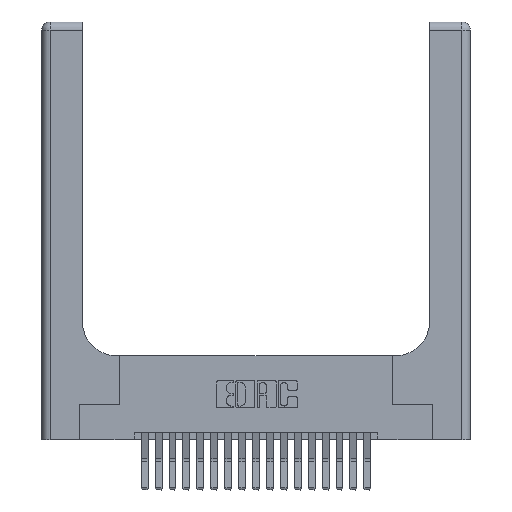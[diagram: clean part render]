
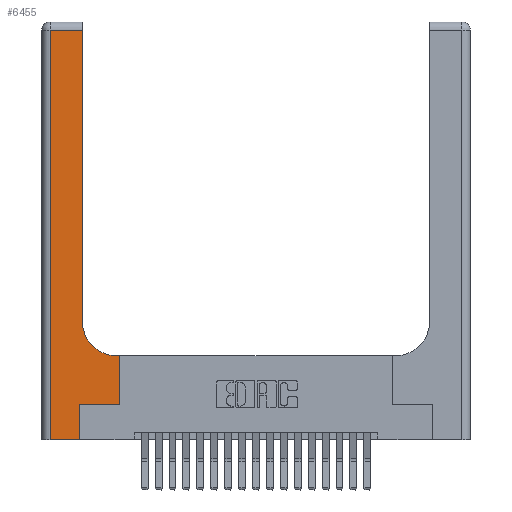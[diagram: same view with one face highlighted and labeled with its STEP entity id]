
A CAD part, top view. The second image highlights one B-rep face of the part: STEP entity #6455.
In plain terms, the highlighted planar face has unit normal (0, 0, 1).
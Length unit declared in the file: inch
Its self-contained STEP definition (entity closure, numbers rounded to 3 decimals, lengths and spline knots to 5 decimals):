
#385 = LINE ( 'NONE', #15664, #17940 ) ;
#422 = LINE ( 'NONE', #11020, #12974 ) ;
#546 = DIRECTION ( 'NONE',  ( 0., -1., 0. ) ) ;
#571 = CARTESIAN_POINT ( 'NONE',  ( 0.06, 3., 0.37 ) ) ;
#1060 = VERTEX_POINT ( 'NONE', #11684 ) ;
#1596 = VECTOR ( 'NONE', #546, 39.37008 ) ;
#1779 = EDGE_CURVE ( 'NONE', #19450, #19559, #10699, .T. ) ;
#1866 = LINE ( 'NONE', #19368, #18860 ) ;
#2386 = DIRECTION ( 'NONE',  ( 0., 1., 0. ) ) ;
#2618 = VERTEX_POINT ( 'NONE', #17655 ) ;
#2654 = VERTEX_POINT ( 'NONE', #4175 ) ;
#2747 = CARTESIAN_POINT ( 'NONE',  ( 0.5415, 0.85, 0.37 ) ) ;
#2955 = CARTESIAN_POINT ( 'NONE',  ( 0.5585, 0.25, 0.37 ) ) ;
#3080 = EDGE_LOOP ( 'NONE', ( #12943, #17093, #20437, #14345, #13760, #20334, #21641, #17208, #16743 ) ) ;
#3719 = AXIS2_PLACEMENT_3D ( 'NONE', #2747, #14628, #4480 ) ;
#4175 = CARTESIAN_POINT ( 'NONE',  ( 0.5585, 0.25, 0.37 ) ) ;
#4232 = DIRECTION ( 'NONE',  ( 0., 1., 0. ) ) ;
#4480 = DIRECTION ( 'NONE',  ( 1., 0., 0. ) ) ;
#4709 = DIRECTION ( 'NONE',  ( 0., 1., 0. ) ) ;
#6141 = CARTESIAN_POINT ( 'NONE',  ( 0.06, 0., 0.37 ) ) ;
#6455 = ADVANCED_FACE ( 'NONE', ( #10802 ), #6953, .F. ) ;
#6487 = LINE ( 'NONE', #2955, #7016 ) ;
#6515 = CARTESIAN_POINT ( 'NONE',  ( 0.2915, 0.6, 0.37 ) ) ;
#6653 = EDGE_CURVE ( 'NONE', #12751, #2654, #20542, .T. ) ;
#6751 = CARTESIAN_POINT ( 'NONE',  ( 0., 0., 0.37 ) ) ;
#6953 = PLANE ( 'NONE',  #19496 ) ;
#7016 = VECTOR ( 'NONE', #4709, 39.37008 ) ;
#7599 = VECTOR ( 'NONE', #19282, 39.37008 ) ;
#8216 = DIRECTION ( 'NONE',  ( -1., 0., 0. ) ) ;
#8656 = DIRECTION ( 'NONE',  ( -1., 0., 0. ) ) ;
#8787 = EDGE_CURVE ( 'NONE', #2654, #1060, #6487, .T. ) ;
#9179 = CARTESIAN_POINT ( 'NONE',  ( 0.269, 0.25, 0.37 ) ) ;
#9576 = VECTOR ( 'NONE', #16884, 39.37008 ) ;
#9809 = EDGE_CURVE ( 'NONE', #10225, #12751, #1866, .T. ) ;
#10061 = VERTEX_POINT ( 'NONE', #18324 ) ;
#10225 = VERTEX_POINT ( 'NONE', #20388 ) ;
#10699 = LINE ( 'NONE', #571, #1596 ) ;
#10802 = FACE_OUTER_BOUND ( 'NONE', #3080, .T. ) ;
#11020 = CARTESIAN_POINT ( 'NONE',  ( 0.2915, 3., 0.37 ) ) ;
#11684 = CARTESIAN_POINT ( 'NONE',  ( 0.5585, 0.6, 0.37 ) ) ;
#12751 = VERTEX_POINT ( 'NONE', #16099 ) ;
#12881 = VECTOR ( 'NONE', #8216, 39.37008 ) ;
#12943 = ORIENTED_EDGE ( 'NONE', *, *, #15789, .T. ) ;
#12974 = VECTOR ( 'NONE', #4232, 39.37008 ) ;
#13684 = CARTESIAN_POINT ( 'NONE',  ( 0., 3., 0.37 ) ) ;
#13760 = ORIENTED_EDGE ( 'NONE', *, *, #9809, .T. ) ;
#14063 = LINE ( 'NONE', #6751, #9576 ) ;
#14345 = ORIENTED_EDGE ( 'NONE', *, *, #14788, .T. ) ;
#14486 = CIRCLE ( 'NONE', #3719, 0.25 ) ;
#14628 = DIRECTION ( 'NONE',  ( 0., 0., -1. ) ) ;
#14788 = EDGE_CURVE ( 'NONE', #19559, #10225, #14063, .T. ) ;
#15664 = CARTESIAN_POINT ( 'NONE',  ( 0., 2.94, 0.37 ) ) ;
#15789 = EDGE_CURVE ( 'NONE', #2618, #15948, #422, .T. ) ;
#15948 = VERTEX_POINT ( 'NONE', #19853 ) ;
#16099 = CARTESIAN_POINT ( 'NONE',  ( 0.269, 0.25, 0.37 ) ) ;
#16743 = ORIENTED_EDGE ( 'NONE', *, *, #17173, .T. ) ;
#16884 = DIRECTION ( 'NONE',  ( 1., 0., 0. ) ) ;
#17093 = ORIENTED_EDGE ( 'NONE', *, *, #19830, .T. ) ;
#17173 = EDGE_CURVE ( 'NONE', #10061, #2618, #14486, .T. ) ;
#17208 = ORIENTED_EDGE ( 'NONE', *, *, #21293, .T. ) ;
#17349 = DIRECTION ( 'NONE',  ( -1., 0., 0. ) ) ;
#17655 = CARTESIAN_POINT ( 'NONE',  ( 0.2915, 0.85, 0.37 ) ) ;
#17743 = CARTESIAN_POINT ( 'NONE',  ( 0.06, 2.94, 0.37 ) ) ;
#17940 = VECTOR ( 'NONE', #17349, 39.37008 ) ;
#18324 = CARTESIAN_POINT ( 'NONE',  ( 0.5415, 0.6, 0.37 ) ) ;
#18770 = DIRECTION ( 'NONE',  ( 0., 0., -1. ) ) ;
#18860 = VECTOR ( 'NONE', #2386, 39.37008 ) ;
#19282 = DIRECTION ( 'NONE',  ( 1., 0., 0. ) ) ;
#19368 = CARTESIAN_POINT ( 'NONE',  ( 0.269, 0., 0.37 ) ) ;
#19450 = VERTEX_POINT ( 'NONE', #17743 ) ;
#19496 = AXIS2_PLACEMENT_3D ( 'NONE', #13684, #18770, #8656 ) ;
#19559 = VERTEX_POINT ( 'NONE', #6141 ) ;
#19830 = EDGE_CURVE ( 'NONE', #15948, #19450, #385, .T. ) ;
#19853 = CARTESIAN_POINT ( 'NONE',  ( 0.2915, 2.94, 0.37 ) ) ;
#20334 = ORIENTED_EDGE ( 'NONE', *, *, #6653, .T. ) ;
#20388 = CARTESIAN_POINT ( 'NONE',  ( 0.269, 0., 0.37 ) ) ;
#20437 = ORIENTED_EDGE ( 'NONE', *, *, #1779, .T. ) ;
#20542 = LINE ( 'NONE', #9179, #7599 ) ;
#21293 = EDGE_CURVE ( 'NONE', #1060, #10061, #21830, .T. ) ;
#21641 = ORIENTED_EDGE ( 'NONE', *, *, #8787, .T. ) ;
#21830 = LINE ( 'NONE', #6515, #12881 ) ;
